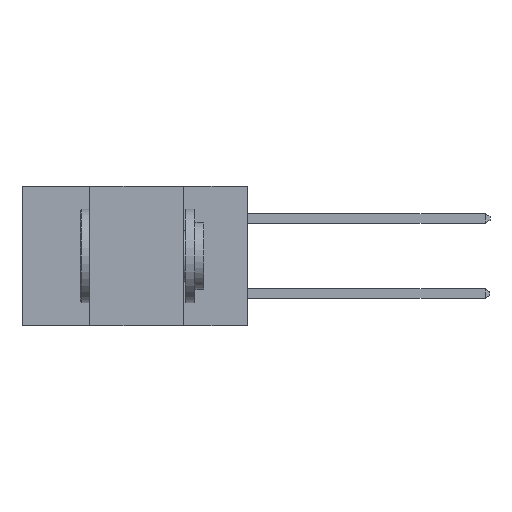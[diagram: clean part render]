
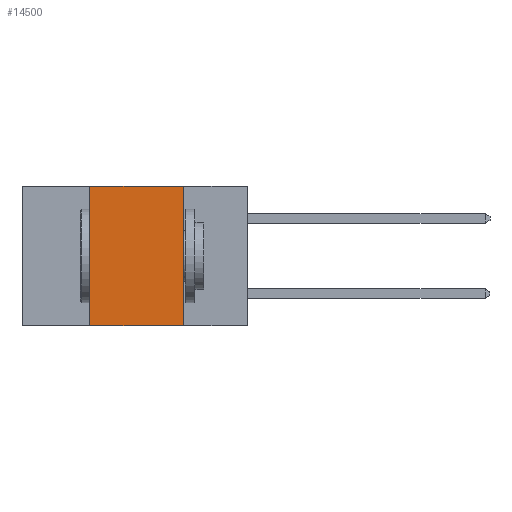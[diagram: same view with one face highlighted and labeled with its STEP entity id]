
A CAD part, left-side view. The second image highlights one B-rep face of the part: STEP entity #14500.
In plain terms, the highlighted planar face has unit normal (-1, 0, 0).
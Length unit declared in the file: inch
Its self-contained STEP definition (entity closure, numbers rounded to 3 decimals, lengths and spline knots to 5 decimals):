
#135 = DIRECTION ( 'NONE',  ( 0., -1., 0. ) ) ;
#409 = AXIS2_PLACEMENT_3D ( 'NONE', #5401, #13518, #6564 ) ;
#1280 = VECTOR ( 'NONE', #10877, 39.37008 ) ;
#1801 = VECTOR ( 'NONE', #135, 39.37008 ) ;
#2231 = FACE_OUTER_BOUND ( 'NONE', #5763, .T. ) ;
#2635 = VECTOR ( 'NONE', #10240, 39.37008 ) ;
#2968 = EDGE_CURVE ( 'NONE', #12886, #14768, #12025, .T. ) ;
#3771 = LINE ( 'NONE', #6209, #12737 ) ;
#5401 = CARTESIAN_POINT ( 'NONE',  ( 0., 0.6, 0. ) ) ;
#5763 = EDGE_LOOP ( 'NONE', ( #6031, #6394, #6782, #7170 ) ) ;
#6031 = ORIENTED_EDGE ( 'NONE', *, *, #7598, .F. ) ;
#6209 = CARTESIAN_POINT ( 'NONE',  ( 0., 0.17, 0. ) ) ;
#6394 = ORIENTED_EDGE ( 'NONE', *, *, #2968, .F. ) ;
#6564 = DIRECTION ( 'NONE',  ( 0., 0., -1. ) ) ;
#6782 = ORIENTED_EDGE ( 'NONE', *, *, #7557, .F. ) ;
#7170 = ORIENTED_EDGE ( 'NONE', *, *, #10823, .T. ) ;
#7243 = VERTEX_POINT ( 'NONE', #13776 ) ;
#7557 = EDGE_CURVE ( 'NONE', #7243, #12886, #8014, .T. ) ;
#7598 = EDGE_CURVE ( 'NONE', #14768, #14546, #3771, .T. ) ;
#7862 = CARTESIAN_POINT ( 'NONE',  ( 0., 0.6, 0. ) ) ;
#8014 = LINE ( 'NONE', #12976, #1280 ) ;
#8579 = DIRECTION ( 'NONE',  ( 0., 0., -1. ) ) ;
#10240 = DIRECTION ( 'NONE',  ( 0., -1., 0. ) ) ;
#10513 = CARTESIAN_POINT ( 'NONE',  ( 0., 0.17, 0. ) ) ;
#10673 = CARTESIAN_POINT ( 'NONE',  ( 0., 0.42, 0. ) ) ;
#10823 = EDGE_CURVE ( 'NONE', #7243, #14546, #11306, .T. ) ;
#10877 = DIRECTION ( 'NONE',  ( 0., 0., 1. ) ) ;
#11306 = LINE ( 'NONE', #12168, #1801 ) ;
#11314 = PLANE ( 'NONE',  #409 ) ;
#12025 = LINE ( 'NONE', #7862, #2635 ) ;
#12168 = CARTESIAN_POINT ( 'NONE',  ( 0., 0.6, -0.37 ) ) ;
#12737 = VECTOR ( 'NONE', #8579, 39.37008 ) ;
#12886 = VERTEX_POINT ( 'NONE', #10673 ) ;
#12976 = CARTESIAN_POINT ( 'NONE',  ( 0., 0.42, 0. ) ) ;
#13518 = DIRECTION ( 'NONE',  ( 1., 0., 0. ) ) ;
#13569 = CARTESIAN_POINT ( 'NONE',  ( 0., 0.17, -0.37 ) ) ;
#13776 = CARTESIAN_POINT ( 'NONE',  ( 0., 0.42, -0.37 ) ) ;
#14500 = ADVANCED_FACE ( 'NONE', ( #2231 ), #11314, .F. ) ;
#14546 = VERTEX_POINT ( 'NONE', #13569 ) ;
#14768 = VERTEX_POINT ( 'NONE', #10513 ) ;
